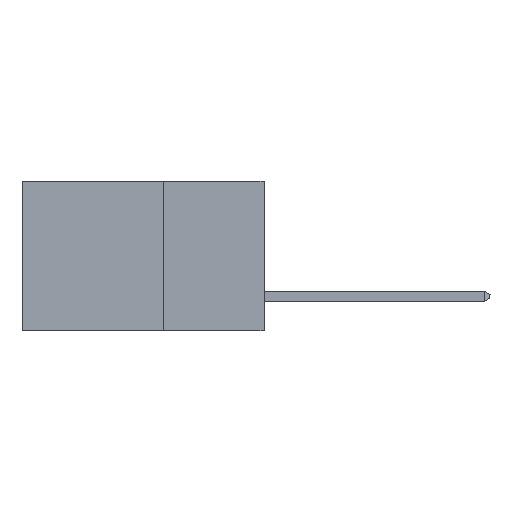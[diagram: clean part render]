
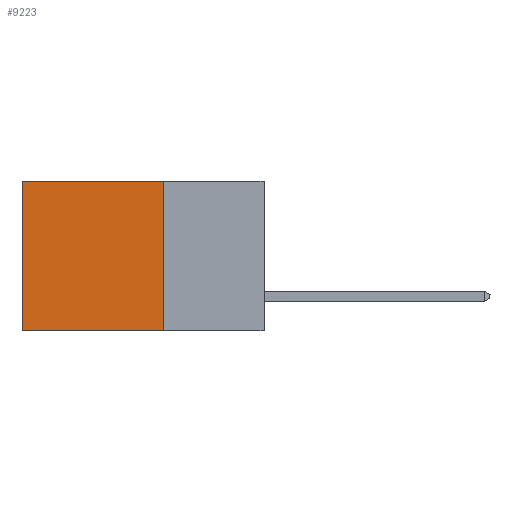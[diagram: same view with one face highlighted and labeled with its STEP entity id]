
A CAD part, left-side view. The second image highlights one B-rep face of the part: STEP entity #9223.
In plain terms, the highlighted planar face has unit normal (-1, 0, 0).
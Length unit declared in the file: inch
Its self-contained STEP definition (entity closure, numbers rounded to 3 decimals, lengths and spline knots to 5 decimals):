
#219 = CARTESIAN_POINT ( 'NONE',  ( 0.298, 0.25, 0. ) ) ;
#401 = VERTEX_POINT ( 'NONE', #11852 ) ;
#636 = ORIENTED_EDGE ( 'NONE', *, *, #16152, .F. ) ;
#1199 = VERTEX_POINT ( 'NONE', #26474 ) ;
#3020 = EDGE_CURVE ( 'NONE', #1199, #401, #13988, .T. ) ;
#3786 = VECTOR ( 'NONE', #31024, 39.37008 ) ;
#4024 = VECTOR ( 'NONE', #11085, 39.37008 ) ;
#4257 = VERTEX_POINT ( 'NONE', #18641 ) ;
#8436 = VERTEX_POINT ( 'NONE', #25108 ) ;
#8808 = EDGE_CURVE ( 'NONE', #8436, #4257, #10343, .T. ) ;
#9223 = ADVANCED_FACE ( 'NONE', ( #26061 ), #25282, .F. ) ;
#10343 = LINE ( 'NONE', #26405, #3786 ) ;
#10604 = CARTESIAN_POINT ( 'NONE',  ( 0.298, 0.25, 0. ) ) ;
#11085 = DIRECTION ( 'NONE',  ( 0., 0., -1. ) ) ;
#11852 = CARTESIAN_POINT ( 'NONE',  ( 0.298, 0.6, 0. ) ) ;
#12863 = EDGE_LOOP ( 'NONE', ( #25254, #20864, #636, #27352 ) ) ;
#13155 = EDGE_CURVE ( 'NONE', #401, #4257, #22859, .T. ) ;
#13253 = DIRECTION ( 'NONE',  ( 0., 1., 0. ) ) ;
#13988 = LINE ( 'NONE', #16050, #17086 ) ;
#16050 = CARTESIAN_POINT ( 'NONE',  ( 0.298, 0.25, 0. ) ) ;
#16152 = EDGE_CURVE ( 'NONE', #1199, #8436, #30209, .T. ) ;
#16798 = VECTOR ( 'NONE', #24996, 39.37008 ) ;
#17086 = VECTOR ( 'NONE', #13253, 39.37008 ) ;
#17535 = AXIS2_PLACEMENT_3D ( 'NONE', #10604, #30252, #25930 ) ;
#18641 = CARTESIAN_POINT ( 'NONE',  ( 0.298, 0.6, -0.37 ) ) ;
#20864 = ORIENTED_EDGE ( 'NONE', *, *, #8808, .F. ) ;
#22859 = LINE ( 'NONE', #25760, #4024 ) ;
#24996 = DIRECTION ( 'NONE',  ( 0., 0., -1. ) ) ;
#25108 = CARTESIAN_POINT ( 'NONE',  ( 0.298, 0.25, -0.37 ) ) ;
#25254 = ORIENTED_EDGE ( 'NONE', *, *, #13155, .T. ) ;
#25282 = PLANE ( 'NONE',  #17535 ) ;
#25760 = CARTESIAN_POINT ( 'NONE',  ( 0.298, 0.6, 0. ) ) ;
#25930 = DIRECTION ( 'NONE',  ( 0., 0., -1. ) ) ;
#26061 = FACE_OUTER_BOUND ( 'NONE', #12863, .T. ) ;
#26405 = CARTESIAN_POINT ( 'NONE',  ( 0.298, 0.25, -0.37 ) ) ;
#26474 = CARTESIAN_POINT ( 'NONE',  ( 0.298, 0.25, 0. ) ) ;
#27352 = ORIENTED_EDGE ( 'NONE', *, *, #3020, .T. ) ;
#30209 = LINE ( 'NONE', #219, #16798 ) ;
#30252 = DIRECTION ( 'NONE',  ( 1., 0., 0. ) ) ;
#31024 = DIRECTION ( 'NONE',  ( 0., 1., 0. ) ) ;
